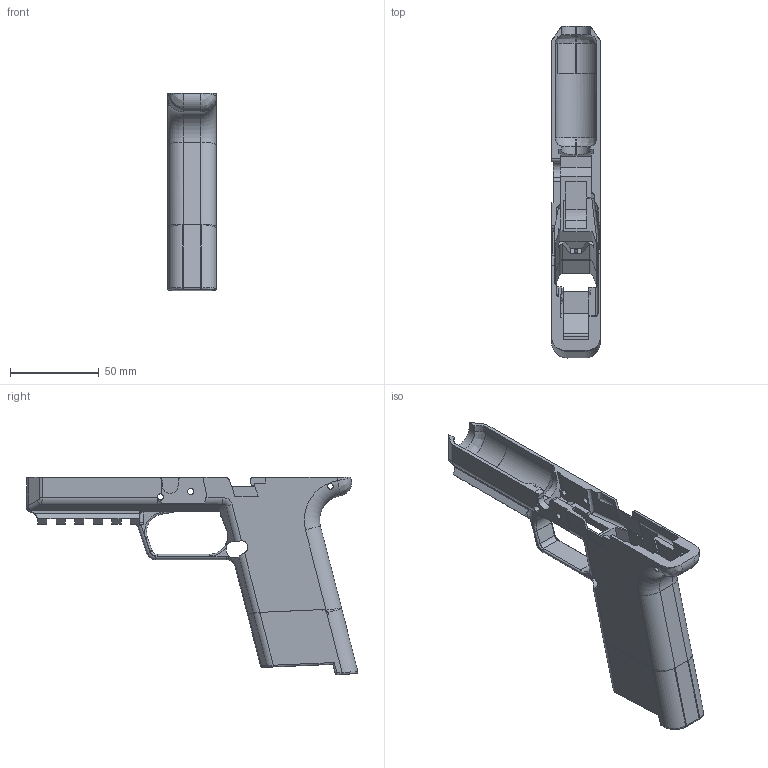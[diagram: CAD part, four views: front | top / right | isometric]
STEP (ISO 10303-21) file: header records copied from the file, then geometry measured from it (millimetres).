
FILE_DESCRIPTION(/* description */ (''),/* implementation_level */ '2;1');
FILE_NAME(/* name */ 'M&P 9 Assembly + Picatinny - Full Size.step',/* time_stamp */ '2021-05-28T01:58:07-04:00',/* author */ (''),/* organization */ (''),/* preprocessor_version */ 'ST-DEVELOPER v18.1',/* originating_system */ 'Autodesk Translation Framework v10.6.0.1341',/* authorisation */ '');
FILE_SCHEMA (('AUTOMOTIVE_DESIGN { 1 0 10303 214 3 1 1 }'));
Length unit declared in the file: millimetre
Products named in the file (6): M&P 9 Standard Length Slide - Picatinny; M&P 9 Reference v87; Frame; Fitment Section; Nose; Full-Size Magwell Body
Assembly tree (5 placements, depth 5):
  M&P 9 Standard Length Slide - Picatinny
    M&P 9 Reference v87
      Frame
        Fitment Section
          Nose
        Full-Size Magwell Body
Bounding box: 27.45 x 187.16 x 111.25 mm (x, y, z)
Volume: 97811.1 mm3; surface area: 50323 mm2
Topology: 4 solids, 4 shells, 444 faces, 1224 edges, 771 vertices
Faces by surface type: plane 213, cylinder 143, bspline 67, torus 14, sphere 6, cone 1
Full cylindrical faces by diameter (mm): 2 x3, 3.18 x2, 3.361 x2, 3.55 x2
Entity records: 16345 total; most frequent: CARTESIAN_POINT 5020, ORIENTED_EDGE 2440, DIRECTION 2249, EDGE_CURVE 1220, VERTEX_POINT 771, AXIS2_PLACEMENT_3D 759, LINE 731, VECTOR 731
